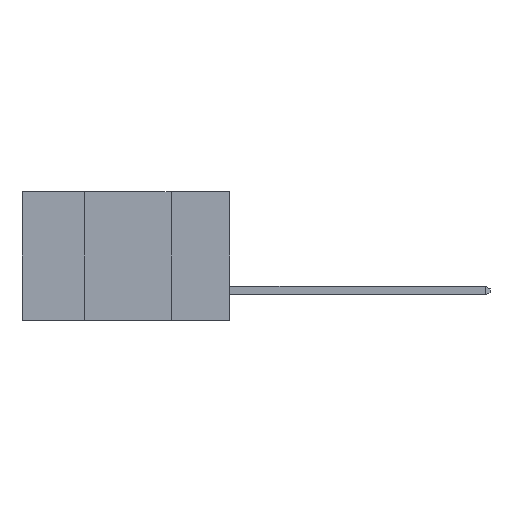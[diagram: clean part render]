
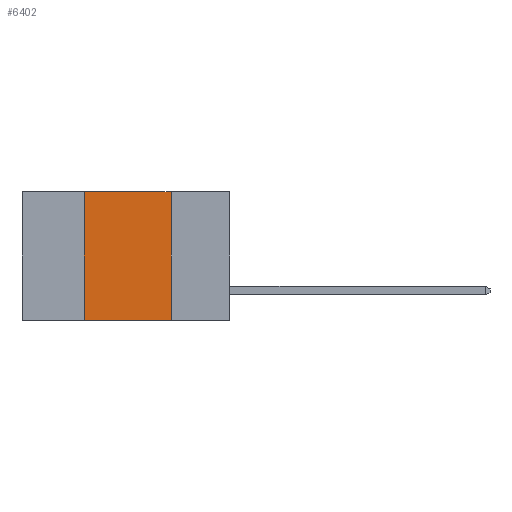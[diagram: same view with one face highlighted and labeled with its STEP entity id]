
A CAD part, left-side view. The second image highlights one B-rep face of the part: STEP entity #6402.
In plain terms, the highlighted planar face has unit normal (-1, 0, 0).
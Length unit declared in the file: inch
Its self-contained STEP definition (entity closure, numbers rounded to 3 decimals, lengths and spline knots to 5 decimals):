
#738 = VECTOR ( 'NONE', #10336, 39.37008 ) ;
#1508 = VERTEX_POINT ( 'NONE', #15138 ) ;
#1548 = LINE ( 'NONE', #3331, #5118 ) ;
#2551 = VECTOR ( 'NONE', #5748, 39.37008 ) ;
#3010 = ORIENTED_EDGE ( 'NONE', *, *, #3608, .T. ) ;
#3331 = CARTESIAN_POINT ( 'NONE',  ( 0., 0.6, 0. ) ) ;
#3536 = FACE_OUTER_BOUND ( 'NONE', #12610, .T. ) ;
#3608 = EDGE_CURVE ( 'NONE', #1508, #12352, #6572, .T. ) ;
#3978 = CARTESIAN_POINT ( 'NONE',  ( 0., 0.6, 0. ) ) ;
#4342 = AXIS2_PLACEMENT_3D ( 'NONE', #3978, #13111, #5307 ) ;
#4514 = EDGE_CURVE ( 'NONE', #1508, #7468, #12217, .T. ) ;
#4673 = DIRECTION ( 'NONE',  ( 0., -1., 0. ) ) ;
#5118 = VECTOR ( 'NONE', #4673, 39.37008 ) ;
#5307 = DIRECTION ( 'NONE',  ( 0., 0., -1. ) ) ;
#5648 = LINE ( 'NONE', #15395, #738 ) ;
#5748 = DIRECTION ( 'NONE',  ( 0., -1., 0. ) ) ;
#6306 = EDGE_CURVE ( 'NONE', #12226, #12352, #5648, .T. ) ;
#6356 = ORIENTED_EDGE ( 'NONE', *, *, #6306, .F. ) ;
#6402 = ADVANCED_FACE ( 'NONE', ( #3536 ), #11820, .F. ) ;
#6572 = LINE ( 'NONE', #7553, #2551 ) ;
#7468 = VERTEX_POINT ( 'NONE', #15480 ) ;
#7553 = CARTESIAN_POINT ( 'NONE',  ( 0., 0.6, -0.37 ) ) ;
#8860 = ORIENTED_EDGE ( 'NONE', *, *, #4514, .F. ) ;
#9202 = CARTESIAN_POINT ( 'NONE',  ( 0., 0.42, 0. ) ) ;
#9219 = VECTOR ( 'NONE', #15557, 39.37008 ) ;
#10336 = DIRECTION ( 'NONE',  ( 0., 0., -1. ) ) ;
#10432 = CARTESIAN_POINT ( 'NONE',  ( 0., 0.17, -0.37 ) ) ;
#11820 = PLANE ( 'NONE',  #4342 ) ;
#12217 = LINE ( 'NONE', #9202, #9219 ) ;
#12226 = VERTEX_POINT ( 'NONE', #16551 ) ;
#12352 = VERTEX_POINT ( 'NONE', #10432 ) ;
#12610 = EDGE_LOOP ( 'NONE', ( #6356, #14047, #8860, #3010 ) ) ;
#13111 = DIRECTION ( 'NONE',  ( 1., 0., 0. ) ) ;
#14047 = ORIENTED_EDGE ( 'NONE', *, *, #14331, .F. ) ;
#14331 = EDGE_CURVE ( 'NONE', #7468, #12226, #1548, .T. ) ;
#15138 = CARTESIAN_POINT ( 'NONE',  ( 0., 0.42, -0.37 ) ) ;
#15395 = CARTESIAN_POINT ( 'NONE',  ( 0., 0.17, 0. ) ) ;
#15480 = CARTESIAN_POINT ( 'NONE',  ( 0., 0.42, 0. ) ) ;
#15557 = DIRECTION ( 'NONE',  ( 0., 0., 1. ) ) ;
#16551 = CARTESIAN_POINT ( 'NONE',  ( 0., 0.17, 0. ) ) ;
